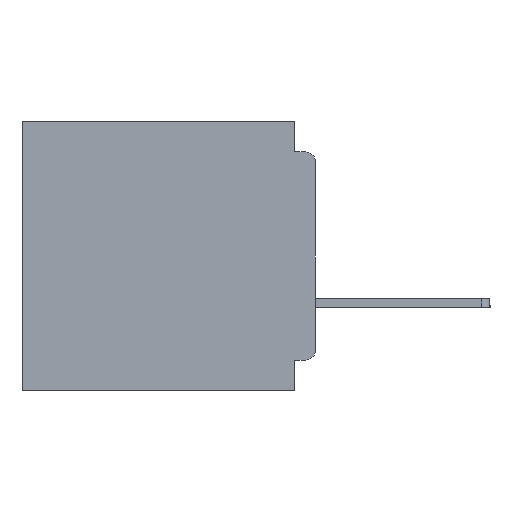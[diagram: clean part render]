
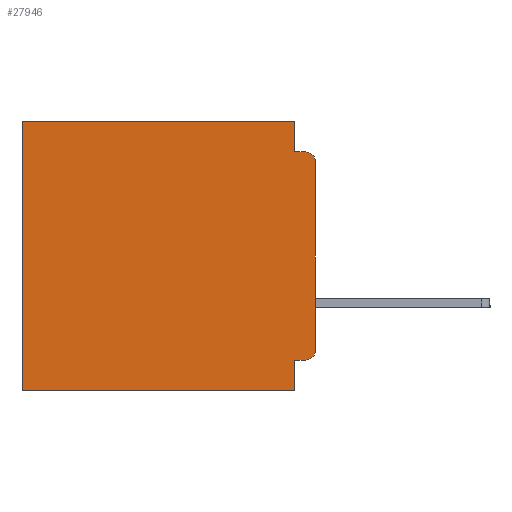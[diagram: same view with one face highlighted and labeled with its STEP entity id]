
A CAD part, left-side view. The second image highlights one B-rep face of the part: STEP entity #27946.
In plain terms, the highlighted planar face has unit normal (-1, 0, 0).
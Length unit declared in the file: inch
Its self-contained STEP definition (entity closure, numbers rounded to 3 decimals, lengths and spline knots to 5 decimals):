
#27 = CARTESIAN_POINT ( 'NONE',  ( 0.3, 0., -0.045 ) ) ;
#412 = VECTOR ( 'NONE', #49320, 39.37008 ) ;
#1099 = VECTOR ( 'NONE', #5782, 39.37008 ) ;
#2254 = DIRECTION ( 'NONE',  ( -1., 0., 0. ) ) ;
#2279 = CIRCLE ( 'NONE', #25057, 0.015 ) ;
#2764 = EDGE_CURVE ( 'NONE', #21594, #32849, #4507, .T. ) ;
#2857 = CARTESIAN_POINT ( 'NONE',  ( 0.3, 0.031, -0.4 ) ) ;
#3635 = EDGE_CURVE ( 'NONE', #19099, #48926, #28377, .T. ) ;
#4066 = FACE_OUTER_BOUND ( 'NONE', #19005, .T. ) ;
#4378 = DIRECTION ( 'NONE',  ( 0., -1., 0. ) ) ;
#4507 = CIRCLE ( 'NONE', #20129, 0.015 ) ;
#5310 = CARTESIAN_POINT ( 'NONE',  ( 0.3, 0.015, -0.045 ) ) ;
#5782 = DIRECTION ( 'NONE',  ( 0., 1., 0. ) ) ;
#6000 = VERTEX_POINT ( 'NONE', #38958 ) ;
#9687 = VERTEX_POINT ( 'NONE', #5310 ) ;
#11894 = CARTESIAN_POINT ( 'NONE',  ( 0.3, 0.031, -0.4 ) ) ;
#11909 = CARTESIAN_POINT ( 'NONE',  ( 0.3, 0., -0.4 ) ) ;
#12029 = CARTESIAN_POINT ( 'NONE',  ( 0.3, 0.015, -0.355 ) ) ;
#12140 = ORIENTED_EDGE ( 'NONE', *, *, #48308, .T. ) ;
#12556 = LINE ( 'NONE', #39932, #1099 ) ;
#12828 = DIRECTION ( 'NONE',  ( 0., 1., 0. ) ) ;
#13918 = ORIENTED_EDGE ( 'NONE', *, *, #19022, .T. ) ;
#14248 = ORIENTED_EDGE ( 'NONE', *, *, #28116, .F. ) ;
#15638 = ORIENTED_EDGE ( 'NONE', *, *, #3635, .F. ) ;
#16153 = LINE ( 'NONE', #27, #37669 ) ;
#16227 = DIRECTION ( 'NONE',  ( 0., 0., -1. ) ) ;
#18516 = VECTOR ( 'NONE', #37815, 39.37008 ) ;
#19005 = EDGE_LOOP ( 'NONE', ( #25952, #32411, #14248, #36574, #12140, #13918, #15638, #54280, #43261, #33467 ) ) ;
#19022 = EDGE_CURVE ( 'NONE', #27389, #48926, #23320, .T. ) ;
#19099 = VERTEX_POINT ( 'NONE', #2857 ) ;
#19833 = EDGE_CURVE ( 'NONE', #21218, #33825, #39935, .T. ) ;
#20129 = AXIS2_PLACEMENT_3D ( 'NONE', #54857, #54350, #28840 ) ;
#20629 = CARTESIAN_POINT ( 'NONE',  ( 0.3, 0.031, -0.045 ) ) ;
#21218 = VERTEX_POINT ( 'NONE', #47828 ) ;
#21594 = VERTEX_POINT ( 'NONE', #12029 ) ;
#21640 = CARTESIAN_POINT ( 'NONE',  ( 0.3, 0.031, 0. ) ) ;
#22971 = VECTOR ( 'NONE', #27933, 39.37008 ) ;
#23320 = LINE ( 'NONE', #49500, #412 ) ;
#24979 = CARTESIAN_POINT ( 'NONE',  ( 0.3, 0., -0.06 ) ) ;
#25057 = AXIS2_PLACEMENT_3D ( 'NONE', #28051, #2254, #32342 ) ;
#25952 = ORIENTED_EDGE ( 'NONE', *, *, #26580, .F. ) ;
#26580 = EDGE_CURVE ( 'NONE', #29090, #32849, #47874, .T. ) ;
#27262 = VECTOR ( 'NONE', #47213, 39.37008 ) ;
#27389 = VERTEX_POINT ( 'NONE', #46416 ) ;
#27933 = DIRECTION ( 'NONE',  ( 0., 1., 0. ) ) ;
#27946 = ADVANCED_FACE ( 'NONE', ( #4066 ), #37653, .F. ) ;
#28051 = CARTESIAN_POINT ( 'NONE',  ( 0.3, 0.015, -0.06 ) ) ;
#28116 = EDGE_CURVE ( 'NONE', #33825, #9687, #16153, .T. ) ;
#28377 = LINE ( 'NONE', #47229, #41047 ) ;
#28840 = DIRECTION ( 'NONE',  ( 0., 0., -1. ) ) ;
#29015 = CARTESIAN_POINT ( 'NONE',  ( 0.3, 0., -0.34 ) ) ;
#29090 = VERTEX_POINT ( 'NONE', #24979 ) ;
#29933 = CARTESIAN_POINT ( 'NONE',  ( 0.3, 0., -0.4 ) ) ;
#30141 = EDGE_CURVE ( 'NONE', #21594, #6000, #12556, .T. ) ;
#31060 = EDGE_CURVE ( 'NONE', #6000, #19099, #52532, .T. ) ;
#31387 = EDGE_CURVE ( 'NONE', #29090, #9687, #2279, .T. ) ;
#32342 = DIRECTION ( 'NONE',  ( 0., 0., -1. ) ) ;
#32411 = ORIENTED_EDGE ( 'NONE', *, *, #31387, .T. ) ;
#32849 = VERTEX_POINT ( 'NONE', #29015 ) ;
#33467 = ORIENTED_EDGE ( 'NONE', *, *, #2764, .T. ) ;
#33825 = VERTEX_POINT ( 'NONE', #20629 ) ;
#34358 = LINE ( 'NONE', #44878, #22971 ) ;
#36574 = ORIENTED_EDGE ( 'NONE', *, *, #19833, .F. ) ;
#36582 = VECTOR ( 'NONE', #55356, 39.37008 ) ;
#37653 = PLANE ( 'NONE',  #45677 ) ;
#37669 = VECTOR ( 'NONE', #4378, 39.37008 ) ;
#37815 = DIRECTION ( 'NONE',  ( 0., 0., -1. ) ) ;
#38958 = CARTESIAN_POINT ( 'NONE',  ( 0.3, 0.031, -0.355 ) ) ;
#39932 = CARTESIAN_POINT ( 'NONE',  ( 0.3, 0., -0.355 ) ) ;
#39935 = LINE ( 'NONE', #21640, #27262 ) ;
#40530 = CARTESIAN_POINT ( 'NONE',  ( 0.3, 0.437, -0.4 ) ) ;
#41047 = VECTOR ( 'NONE', #12828, 39.37008 ) ;
#41867 = DIRECTION ( 'NONE',  ( 1., 0., 0. ) ) ;
#43261 = ORIENTED_EDGE ( 'NONE', *, *, #30141, .F. ) ;
#44878 = CARTESIAN_POINT ( 'NONE',  ( 0.3, 0., 0. ) ) ;
#45677 = AXIS2_PLACEMENT_3D ( 'NONE', #11909, #41867, #16227 ) ;
#46416 = CARTESIAN_POINT ( 'NONE',  ( 0.3, 0.437, 0. ) ) ;
#47213 = DIRECTION ( 'NONE',  ( 0., 0., -1. ) ) ;
#47229 = CARTESIAN_POINT ( 'NONE',  ( 0.3, 0., -0.4 ) ) ;
#47828 = CARTESIAN_POINT ( 'NONE',  ( 0.3, 0.031, 0. ) ) ;
#47874 = LINE ( 'NONE', #29933, #36582 ) ;
#48308 = EDGE_CURVE ( 'NONE', #21218, #27389, #34358, .T. ) ;
#48926 = VERTEX_POINT ( 'NONE', #40530 ) ;
#49320 = DIRECTION ( 'NONE',  ( 0., 0., -1. ) ) ;
#49500 = CARTESIAN_POINT ( 'NONE',  ( 0.3, 0.437, -0.4 ) ) ;
#52532 = LINE ( 'NONE', #11894, #18516 ) ;
#54280 = ORIENTED_EDGE ( 'NONE', *, *, #31060, .F. ) ;
#54350 = DIRECTION ( 'NONE',  ( -1., 0., 0. ) ) ;
#54857 = CARTESIAN_POINT ( 'NONE',  ( 0.3, 0.015, -0.34 ) ) ;
#55356 = DIRECTION ( 'NONE',  ( 0., 0., -1. ) ) ;
